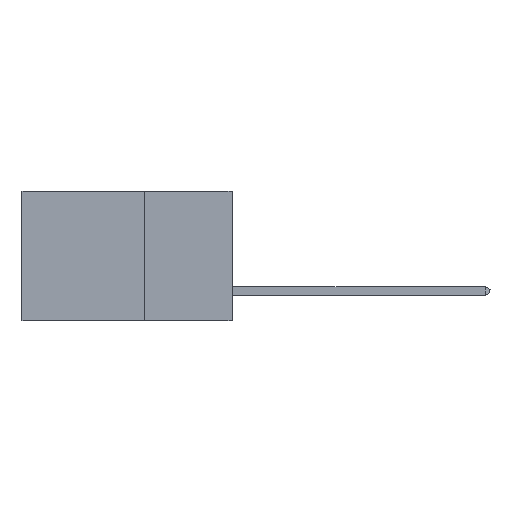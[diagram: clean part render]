
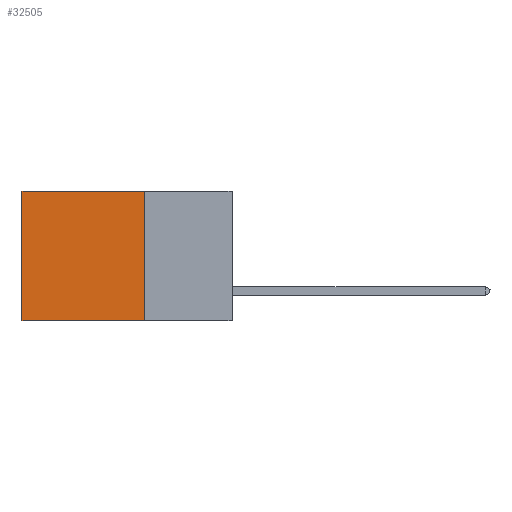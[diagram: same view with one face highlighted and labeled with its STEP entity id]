
A CAD part, left-side view. The second image highlights one B-rep face of the part: STEP entity #32505.
In plain terms, the highlighted planar face has unit normal (-1, 0, 0).
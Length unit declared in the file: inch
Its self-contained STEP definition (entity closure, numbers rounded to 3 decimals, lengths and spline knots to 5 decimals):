
#3229 = VERTEX_POINT ( 'NONE', #24904 ) ;
#3518 = VECTOR ( 'NONE', #44087, 39.37008 ) ;
#4221 = LINE ( 'NONE', #5265, #41999 ) ;
#4562 = AXIS2_PLACEMENT_3D ( 'NONE', #35208, #5767, #42408 ) ;
#5265 = CARTESIAN_POINT ( 'NONE',  ( 0.2875, 0.6, 0. ) ) ;
#5444 = EDGE_CURVE ( 'NONE', #43580, #42509, #9013, .T. ) ;
#5767 = DIRECTION ( 'NONE',  ( 1., 0., 0. ) ) ;
#6913 = VECTOR ( 'NONE', #25891, 39.37008 ) ;
#7465 = EDGE_CURVE ( 'NONE', #3229, #42509, #4221, .T. ) ;
#8995 = ORIENTED_EDGE ( 'NONE', *, *, #7465, .T. ) ;
#9013 = LINE ( 'NONE', #17262, #45656 ) ;
#9174 = ORIENTED_EDGE ( 'NONE', *, *, #5444, .F. ) ;
#9183 = LINE ( 'NONE', #29563, #6913 ) ;
#9589 = ORIENTED_EDGE ( 'NONE', *, *, #17975, .F. ) ;
#12980 = EDGE_CURVE ( 'NONE', #31497, #3229, #9183, .T. ) ;
#13844 = CARTESIAN_POINT ( 'NONE',  ( 0.2875, 0.25, 0. ) ) ;
#17262 = CARTESIAN_POINT ( 'NONE',  ( 0.2875, 0.25, -0.37 ) ) ;
#17975 = EDGE_CURVE ( 'NONE', #31497, #43580, #43609, .T. ) ;
#19812 = EDGE_LOOP ( 'NONE', ( #8995, #9174, #9589, #37338 ) ) ;
#24483 = PLANE ( 'NONE',  #4562 ) ;
#24904 = CARTESIAN_POINT ( 'NONE',  ( 0.2875, 0.6, 0. ) ) ;
#25891 = DIRECTION ( 'NONE',  ( 0., 1., 0. ) ) ;
#29516 = CARTESIAN_POINT ( 'NONE',  ( 0.2875, 0.25, 0. ) ) ;
#29563 = CARTESIAN_POINT ( 'NONE',  ( 0.2875, 0.25, 0. ) ) ;
#29935 = CARTESIAN_POINT ( 'NONE',  ( 0.2875, 0.6, -0.37 ) ) ;
#31497 = VERTEX_POINT ( 'NONE', #13844 ) ;
#32505 = ADVANCED_FACE ( 'NONE', ( #35518 ), #24483, .F. ) ;
#35208 = CARTESIAN_POINT ( 'NONE',  ( 0.2875, 0.25, 0. ) ) ;
#35518 = FACE_OUTER_BOUND ( 'NONE', #19812, .T. ) ;
#37338 = ORIENTED_EDGE ( 'NONE', *, *, #12980, .T. ) ;
#39187 = DIRECTION ( 'NONE',  ( 0., 1., 0. ) ) ;
#39771 = CARTESIAN_POINT ( 'NONE',  ( 0.2875, 0.25, -0.37 ) ) ;
#41999 = VECTOR ( 'NONE', #42058, 39.37008 ) ;
#42058 = DIRECTION ( 'NONE',  ( 0., 0., -1. ) ) ;
#42408 = DIRECTION ( 'NONE',  ( 0., 0., -1. ) ) ;
#42509 = VERTEX_POINT ( 'NONE', #29935 ) ;
#43580 = VERTEX_POINT ( 'NONE', #39771 ) ;
#43609 = LINE ( 'NONE', #29516, #3518 ) ;
#44087 = DIRECTION ( 'NONE',  ( 0., 0., -1. ) ) ;
#45656 = VECTOR ( 'NONE', #39187, 39.37008 ) ;
